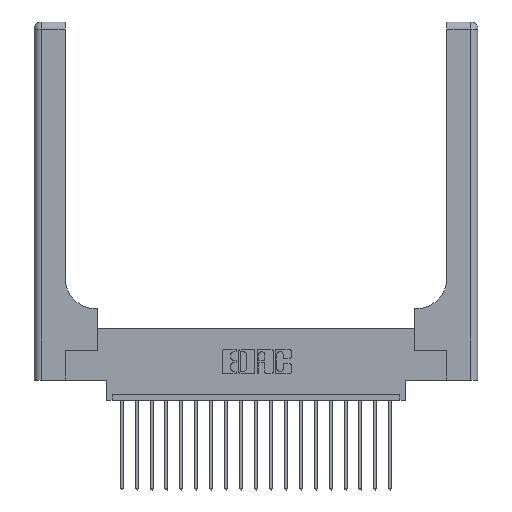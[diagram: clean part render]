
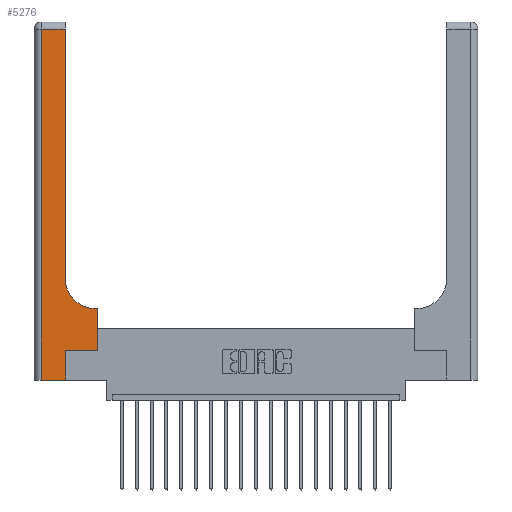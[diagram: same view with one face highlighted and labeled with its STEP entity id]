
A CAD part, top view. The second image highlights one B-rep face of the part: STEP entity #5276.
In plain terms, the highlighted planar face has unit normal (0, 0, 1).
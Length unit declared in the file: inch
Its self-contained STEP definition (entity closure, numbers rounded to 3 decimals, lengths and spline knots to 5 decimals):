
#584 = CARTESIAN_POINT ( 'NONE',  ( 0.528, 0.25, 0.37 ) ) ;
#694 = VECTOR ( 'NONE', #8828, 39.37008 ) ;
#1046 = DIRECTION ( 'NONE',  ( 0., 1., 0. ) ) ;
#1107 = EDGE_CURVE ( 'NONE', #2944, #10689, #9638, .T. ) ;
#1184 = LINE ( 'NONE', #5912, #3105 ) ;
#1281 = ORIENTED_EDGE ( 'NONE', *, *, #11105, .T. ) ;
#2175 = CARTESIAN_POINT ( 'NONE',  ( 0., 3., 0.37 ) ) ;
#2453 = ORIENTED_EDGE ( 'NONE', *, *, #5859, .T. ) ;
#2512 = EDGE_CURVE ( 'NONE', #7512, #13035, #14237, .T. ) ;
#2944 = VERTEX_POINT ( 'NONE', #11512 ) ;
#3048 = CARTESIAN_POINT ( 'NONE',  ( 0.06, 0., 0.37 ) ) ;
#3105 = VECTOR ( 'NONE', #12063, 39.37008 ) ;
#4162 = LINE ( 'NONE', #16288, #11502 ) ;
#4215 = CARTESIAN_POINT ( 'NONE',  ( 0.51, 0.85, 0.37 ) ) ;
#4477 = CARTESIAN_POINT ( 'NONE',  ( 0.528, 0.6, 0.37 ) ) ;
#4591 = VERTEX_POINT ( 'NONE', #7960 ) ;
#4719 = DIRECTION ( 'NONE',  ( 0., -1., 0. ) ) ;
#5197 = CARTESIAN_POINT ( 'NONE',  ( 0.26, 0.6, 0.37 ) ) ;
#5276 = ADVANCED_FACE ( 'NONE', ( #5551 ), #17860, .F. ) ;
#5406 = CARTESIAN_POINT ( 'NONE',  ( 0.51, 0.6, 0.37 ) ) ;
#5551 = FACE_OUTER_BOUND ( 'NONE', #9190, .T. ) ;
#5585 = CIRCLE ( 'NONE', #17491, 0.25 ) ;
#5859 = EDGE_CURVE ( 'NONE', #10689, #9633, #6009, .T. ) ;
#5912 = CARTESIAN_POINT ( 'NONE',  ( 0.265, 0.25, 0.37 ) ) ;
#5949 = CARTESIAN_POINT ( 'NONE',  ( 0., 0., 0.37 ) ) ;
#6009 = LINE ( 'NONE', #5949, #11633 ) ;
#7061 = ORIENTED_EDGE ( 'NONE', *, *, #1107, .T. ) ;
#7404 = CARTESIAN_POINT ( 'NONE',  ( 0.265, 0., 0.37 ) ) ;
#7512 = VERTEX_POINT ( 'NONE', #584 ) ;
#7894 = CARTESIAN_POINT ( 'NONE',  ( 0.265, 0., 0.37 ) ) ;
#7960 = CARTESIAN_POINT ( 'NONE',  ( 0.265, 0.25, 0.37 ) ) ;
#8260 = DIRECTION ( 'NONE',  ( -1., 0., 0. ) ) ;
#8786 = AXIS2_PLACEMENT_3D ( 'NONE', #2175, #16115, #19466 ) ;
#8828 = DIRECTION ( 'NONE',  ( 0., 1., 0. ) ) ;
#8945 = DIRECTION ( 'NONE',  ( 0., 0., -1. ) ) ;
#8950 = CARTESIAN_POINT ( 'NONE',  ( 0.26, 0.85, 0.37 ) ) ;
#9035 = CARTESIAN_POINT ( 'NONE',  ( 0.528, 0.25, 0.37 ) ) ;
#9063 = EDGE_CURVE ( 'NONE', #10269, #2944, #4162, .T. ) ;
#9136 = ORIENTED_EDGE ( 'NONE', *, *, #13532, .T. ) ;
#9190 = EDGE_LOOP ( 'NONE', ( #9136, #16937, #7061, #2453, #1281, #12103, #13684, #14115, #18610 ) ) ;
#9346 = VECTOR ( 'NONE', #1046, 39.37008 ) ;
#9633 = VERTEX_POINT ( 'NONE', #7894 ) ;
#9638 = LINE ( 'NONE', #18605, #11595 ) ;
#9905 = VERTEX_POINT ( 'NONE', #5406 ) ;
#10269 = VERTEX_POINT ( 'NONE', #19023 ) ;
#10631 = EDGE_CURVE ( 'NONE', #9905, #11522, #5585, .T. ) ;
#10689 = VERTEX_POINT ( 'NONE', #3048 ) ;
#11105 = EDGE_CURVE ( 'NONE', #9633, #4591, #18287, .T. ) ;
#11502 = VECTOR ( 'NONE', #11640, 39.37008 ) ;
#11512 = CARTESIAN_POINT ( 'NONE',  ( 0.06, 2.94, 0.37 ) ) ;
#11517 = EDGE_CURVE ( 'NONE', #13035, #9905, #14715, .T. ) ;
#11522 = VERTEX_POINT ( 'NONE', #8950 ) ;
#11595 = VECTOR ( 'NONE', #4719, 39.37008 ) ;
#11633 = VECTOR ( 'NONE', #18457, 39.37008 ) ;
#11640 = DIRECTION ( 'NONE',  ( -1., 0., 0. ) ) ;
#12063 = DIRECTION ( 'NONE',  ( 1., 0., 0. ) ) ;
#12103 = ORIENTED_EDGE ( 'NONE', *, *, #18373, .T. ) ;
#13035 = VERTEX_POINT ( 'NONE', #4477 ) ;
#13532 = EDGE_CURVE ( 'NONE', #11522, #10269, #17234, .T. ) ;
#13684 = ORIENTED_EDGE ( 'NONE', *, *, #2512, .T. ) ;
#13997 = VECTOR ( 'NONE', #8260, 39.37008 ) ;
#14066 = VECTOR ( 'NONE', #14938, 39.37008 ) ;
#14115 = ORIENTED_EDGE ( 'NONE', *, *, #11517, .T. ) ;
#14237 = LINE ( 'NONE', #9035, #9346 ) ;
#14715 = LINE ( 'NONE', #5197, #13997 ) ;
#14938 = DIRECTION ( 'NONE',  ( 0., 1., 0. ) ) ;
#16115 = DIRECTION ( 'NONE',  ( 0., 0., -1. ) ) ;
#16288 = CARTESIAN_POINT ( 'NONE',  ( 0., 2.94, 0.37 ) ) ;
#16937 = ORIENTED_EDGE ( 'NONE', *, *, #9063, .T. ) ;
#17234 = LINE ( 'NONE', #17999, #14066 ) ;
#17491 = AXIS2_PLACEMENT_3D ( 'NONE', #4215, #8945, #19886 ) ;
#17860 = PLANE ( 'NONE',  #8786 ) ;
#17999 = CARTESIAN_POINT ( 'NONE',  ( 0.26, 3., 0.37 ) ) ;
#18287 = LINE ( 'NONE', #7404, #694 ) ;
#18373 = EDGE_CURVE ( 'NONE', #4591, #7512, #1184, .T. ) ;
#18457 = DIRECTION ( 'NONE',  ( 1., 0., 0. ) ) ;
#18605 = CARTESIAN_POINT ( 'NONE',  ( 0.06, 3., 0.37 ) ) ;
#18610 = ORIENTED_EDGE ( 'NONE', *, *, #10631, .T. ) ;
#19023 = CARTESIAN_POINT ( 'NONE',  ( 0.26, 2.94, 0.37 ) ) ;
#19466 = DIRECTION ( 'NONE',  ( -1., 0., 0. ) ) ;
#19886 = DIRECTION ( 'NONE',  ( 1., 0., 0. ) ) ;
